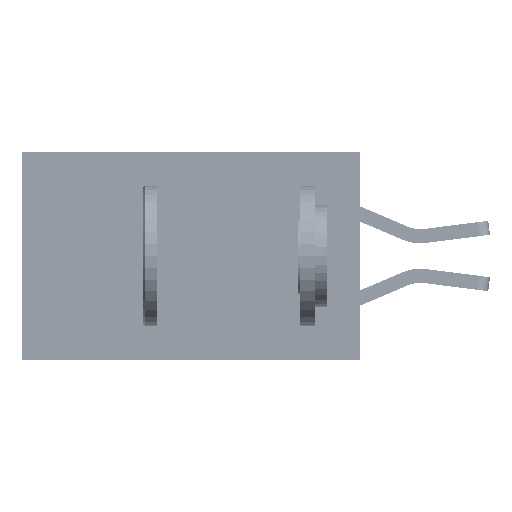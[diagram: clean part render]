
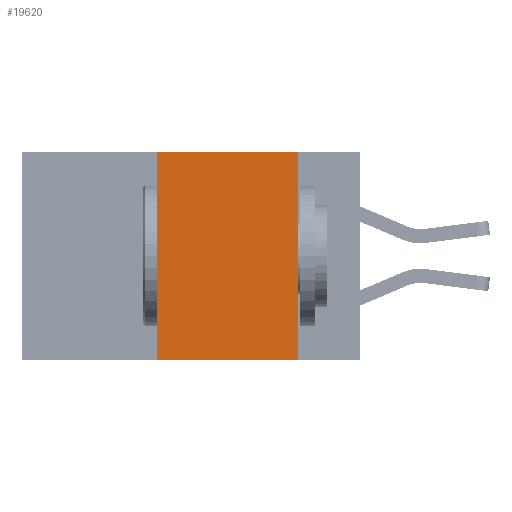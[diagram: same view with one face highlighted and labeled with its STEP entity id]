
A CAD part, left-side view. The second image highlights one B-rep face of the part: STEP entity #19620.
In plain terms, the highlighted planar face has unit normal (-1, 0, 0).
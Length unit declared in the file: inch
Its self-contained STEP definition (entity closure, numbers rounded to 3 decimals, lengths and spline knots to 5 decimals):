
#692 = DIRECTION ( 'NONE',  ( 0., 0., 1. ) ) ;
#1428 = ORIENTED_EDGE ( 'NONE', *, *, #15036, .T. ) ;
#1861 = EDGE_CURVE ( 'NONE', #12066, #28709, #31919, .T. ) ;
#4046 = VECTOR ( 'NONE', #30069, 39.37008 ) ;
#4617 = LINE ( 'NONE', #12336, #20186 ) ;
#5058 = DIRECTION ( 'NONE',  ( 0., -1., 0. ) ) ;
#5483 = EDGE_CURVE ( 'NONE', #36613, #12066, #33846, .T. ) ;
#7640 = CARTESIAN_POINT ( 'NONE',  ( 0., 0.6, 0. ) ) ;
#9036 = EDGE_LOOP ( 'NONE', ( #27516, #26431, #17606, #1428 ) ) ;
#9556 = CARTESIAN_POINT ( 'NONE',  ( 0., 0.11, 0. ) ) ;
#11881 = VECTOR ( 'NONE', #692, 39.37008 ) ;
#12066 = VERTEX_POINT ( 'NONE', #23591 ) ;
#12336 = CARTESIAN_POINT ( 'NONE',  ( 0., 0.6, -0.37 ) ) ;
#13675 = DIRECTION ( 'NONE',  ( 1., 0., 0. ) ) ;
#15036 = EDGE_CURVE ( 'NONE', #29107, #28709, #4617, .T. ) ;
#15293 = CARTESIAN_POINT ( 'NONE',  ( 0., 0.36, 0. ) ) ;
#15524 = EDGE_CURVE ( 'NONE', #29107, #36613, #25681, .T. ) ;
#16120 = CARTESIAN_POINT ( 'NONE',  ( 0., 0.36, -0.37 ) ) ;
#16350 = DIRECTION ( 'NONE',  ( 0., 0., -1. ) ) ;
#17606 = ORIENTED_EDGE ( 'NONE', *, *, #15524, .F. ) ;
#18700 = AXIS2_PLACEMENT_3D ( 'NONE', #7640, #13675, #16350 ) ;
#19620 = ADVANCED_FACE ( 'NONE', ( #20689 ), #31366, .F. ) ;
#19995 = CARTESIAN_POINT ( 'NONE',  ( 0., 0.11, -0.37 ) ) ;
#20186 = VECTOR ( 'NONE', #27226, 39.37008 ) ;
#20689 = FACE_OUTER_BOUND ( 'NONE', #9036, .T. ) ;
#21460 = VECTOR ( 'NONE', #5058, 39.37008 ) ;
#23591 = CARTESIAN_POINT ( 'NONE',  ( 0., 0.11, 0. ) ) ;
#25681 = LINE ( 'NONE', #15293, #11881 ) ;
#26431 = ORIENTED_EDGE ( 'NONE', *, *, #5483, .F. ) ;
#27226 = DIRECTION ( 'NONE',  ( 0., -1., 0. ) ) ;
#27516 = ORIENTED_EDGE ( 'NONE', *, *, #1861, .F. ) ;
#28709 = VERTEX_POINT ( 'NONE', #19995 ) ;
#29107 = VERTEX_POINT ( 'NONE', #16120 ) ;
#29967 = CARTESIAN_POINT ( 'NONE',  ( 0., 0.36, 0. ) ) ;
#30069 = DIRECTION ( 'NONE',  ( 0., 0., -1. ) ) ;
#31366 = PLANE ( 'NONE',  #18700 ) ;
#31919 = LINE ( 'NONE', #9556, #4046 ) ;
#33846 = LINE ( 'NONE', #34136, #21460 ) ;
#34136 = CARTESIAN_POINT ( 'NONE',  ( 0., 0.6, 0. ) ) ;
#36613 = VERTEX_POINT ( 'NONE', #29967 ) ;
